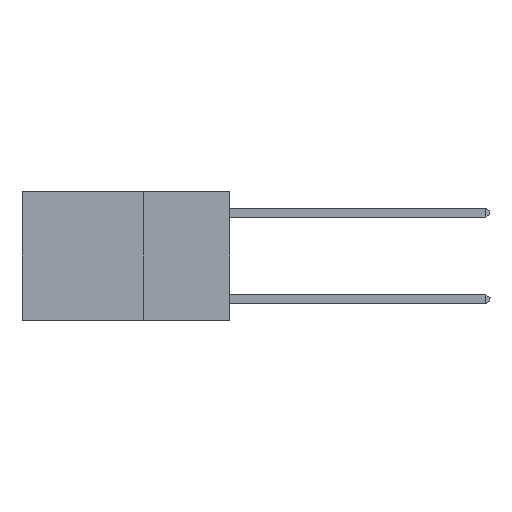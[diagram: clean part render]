
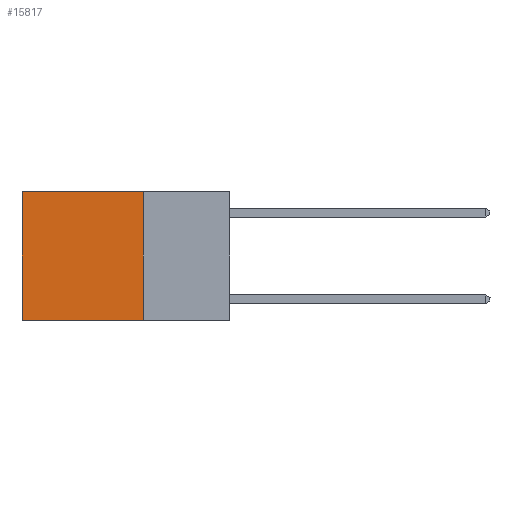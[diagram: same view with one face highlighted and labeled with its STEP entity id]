
A CAD part, left-side view. The second image highlights one B-rep face of the part: STEP entity #15817.
In plain terms, the highlighted planar face has unit normal (-1, 0, 0).
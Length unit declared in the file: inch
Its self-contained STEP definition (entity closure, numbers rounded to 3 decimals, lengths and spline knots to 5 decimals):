
#680 = EDGE_LOOP ( 'NONE', ( #9532, #17790, #12488, #8070 ) ) ;
#706 = EDGE_CURVE ( 'NONE', #24524, #8378, #4755, .T. ) ;
#1855 = LINE ( 'NONE', #3375, #20238 ) ;
#3375 = CARTESIAN_POINT ( 'NONE',  ( 0.2625, 0.25, -0.37 ) ) ;
#3540 = VERTEX_POINT ( 'NONE', #20825 ) ;
#4755 = LINE ( 'NONE', #23699, #20106 ) ;
#6834 = VECTOR ( 'NONE', #20362, 39.37008 ) ;
#7509 = DIRECTION ( 'NONE',  ( 0., 1., 0. ) ) ;
#7919 = FACE_OUTER_BOUND ( 'NONE', #680, .T. ) ;
#8070 = ORIENTED_EDGE ( 'NONE', *, *, #21837, .T. ) ;
#8378 = VERTEX_POINT ( 'NONE', #12892 ) ;
#9532 = ORIENTED_EDGE ( 'NONE', *, *, #706, .T. ) ;
#9566 = CARTESIAN_POINT ( 'NONE',  ( 0.2625, 0.25, -0.37 ) ) ;
#9870 = VECTOR ( 'NONE', #22044, 39.37008 ) ;
#10409 = DIRECTION ( 'NONE',  ( 1., 0., 0. ) ) ;
#12488 = ORIENTED_EDGE ( 'NONE', *, *, #14985, .F. ) ;
#12784 = EDGE_CURVE ( 'NONE', #18706, #8378, #1855, .T. ) ;
#12892 = CARTESIAN_POINT ( 'NONE',  ( 0.2625, 0.6, -0.37 ) ) ;
#14985 = EDGE_CURVE ( 'NONE', #3540, #18706, #20403, .T. ) ;
#15817 = ADVANCED_FACE ( 'NONE', ( #7919 ), #19693, .F. ) ;
#16319 = LINE ( 'NONE', #23989, #6834 ) ;
#17356 = AXIS2_PLACEMENT_3D ( 'NONE', #17936, #10409, #18058 ) ;
#17790 = ORIENTED_EDGE ( 'NONE', *, *, #12784, .F. ) ;
#17936 = CARTESIAN_POINT ( 'NONE',  ( 0.2625, 0.25, 0. ) ) ;
#18058 = DIRECTION ( 'NONE',  ( 0., 0., -1. ) ) ;
#18706 = VERTEX_POINT ( 'NONE', #9566 ) ;
#19693 = PLANE ( 'NONE',  #17356 ) ;
#20106 = VECTOR ( 'NONE', #24288, 39.37008 ) ;
#20238 = VECTOR ( 'NONE', #7509, 39.37008 ) ;
#20362 = DIRECTION ( 'NONE',  ( 0., 1., 0. ) ) ;
#20403 = LINE ( 'NONE', #23659, #9870 ) ;
#20825 = CARTESIAN_POINT ( 'NONE',  ( 0.2625, 0.25, 0. ) ) ;
#21837 = EDGE_CURVE ( 'NONE', #3540, #24524, #16319, .T. ) ;
#22044 = DIRECTION ( 'NONE',  ( 0., 0., -1. ) ) ;
#22384 = CARTESIAN_POINT ( 'NONE',  ( 0.2625, 0.6, 0. ) ) ;
#23659 = CARTESIAN_POINT ( 'NONE',  ( 0.2625, 0.25, 0. ) ) ;
#23699 = CARTESIAN_POINT ( 'NONE',  ( 0.2625, 0.6, 0. ) ) ;
#23989 = CARTESIAN_POINT ( 'NONE',  ( 0.2625, 0.25, 0. ) ) ;
#24288 = DIRECTION ( 'NONE',  ( 0., 0., -1. ) ) ;
#24524 = VERTEX_POINT ( 'NONE', #22384 ) ;
